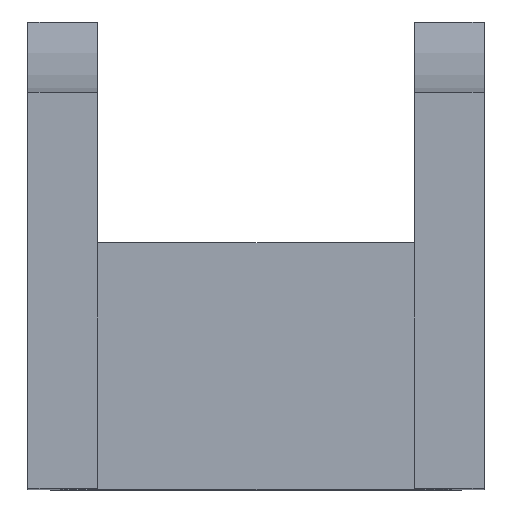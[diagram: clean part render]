
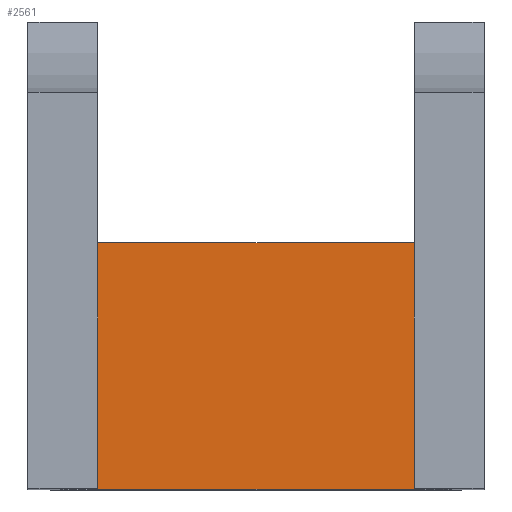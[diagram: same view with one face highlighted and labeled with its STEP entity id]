
A CAD part, top view. The second image highlights one B-rep face of the part: STEP entity #2561.
In plain terms, the highlighted planar face has unit normal (0, 0, 1).
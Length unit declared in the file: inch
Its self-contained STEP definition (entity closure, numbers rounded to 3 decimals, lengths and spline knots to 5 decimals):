
#46=PLANE('',#2736);
#185=FACE_OUTER_BOUND('',#332,.T.);
#332=EDGE_LOOP('',(#2284,#2285,#2286,#2287));
#699=LINE('',#7900,#839);
#710=LINE('',#9979,#850);
#717=LINE('',#10009,#857);
#734=LINE('',#10113,#874);
#839=VECTOR('',#3085,0.3937);
#850=VECTOR('',#3112,0.3937);
#857=VECTOR('',#3129,0.3937);
#874=VECTOR('',#3196,0.3937);
#1104=VERTEX_POINT('',#7898);
#1105=VERTEX_POINT('',#7899);
#1115=VERTEX_POINT('',#9978);
#1125=VERTEX_POINT('',#10008);
#1470=EDGE_CURVE('',#1104,#1105,#699,.T.);
#1489=EDGE_CURVE('',#1115,#1105,#710,.T.);
#1502=EDGE_CURVE('',#1104,#1125,#717,.T.);
#1530=EDGE_CURVE('',#1115,#1125,#734,.T.);
#2284=ORIENTED_EDGE('',*,*,#1530,.T.);
#2285=ORIENTED_EDGE('',*,*,#1502,.F.);
#2286=ORIENTED_EDGE('',*,*,#1470,.T.);
#2287=ORIENTED_EDGE('',*,*,#1489,.F.);
#2561=ADVANCED_FACE('',(#185),#46,.T.);
#2736=AXIS2_PLACEMENT_3D('',#10112,#3194,#3195);
#3085=DIRECTION('',(0.,-1.,0.));
#3112=DIRECTION('',(-1.,0.,0.));
#3129=DIRECTION('',(1.,0.,0.));
#3194=DIRECTION('center_axis',(0.,0.,1.));
#3195=DIRECTION('ref_axis',(0.,1.,0.));
#3196=DIRECTION('',(0.,1.,0.));
#7898=CARTESIAN_POINT('',(-0.252,-0.238,-3.382));
#7899=CARTESIAN_POINT('',(-0.252,-0.63,-3.382));
#7900=CARTESIAN_POINT('',(-0.252,-0.4725,-3.382));
#9978=CARTESIAN_POINT('',(0.252,-0.63,-3.382));
#9979=CARTESIAN_POINT('',(-0.0705,-0.63,-3.382));
#10008=CARTESIAN_POINT('',(0.252,-0.238,-3.382));
#10009=CARTESIAN_POINT('',(0.,-0.238,-3.382));
#10112=CARTESIAN_POINT('Origin',(0.,-0.63,-3.382));
#10113=CARTESIAN_POINT('',(0.252,-0.4725,-3.382));
